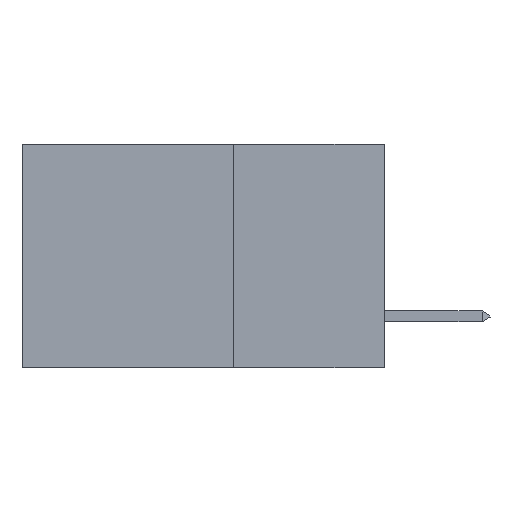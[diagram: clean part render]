
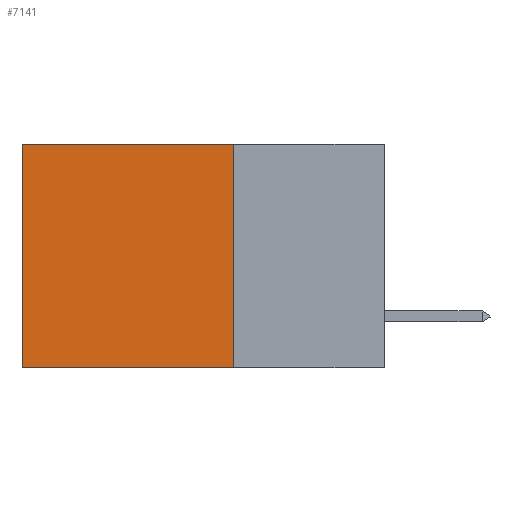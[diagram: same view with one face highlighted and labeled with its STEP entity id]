
A CAD part, left-side view. The second image highlights one B-rep face of the part: STEP entity #7141.
In plain terms, the highlighted planar face has unit normal (-1, 0, 0).
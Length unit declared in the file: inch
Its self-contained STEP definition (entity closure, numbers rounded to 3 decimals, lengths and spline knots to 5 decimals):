
#750 = DIRECTION ( 'NONE',  ( 0., 1., 0. ) ) ;
#767 = CARTESIAN_POINT ( 'NONE',  ( 0.2875, 0.25, 0. ) ) ;
#786 = CARTESIAN_POINT ( 'NONE',  ( 0.2875, 0.25, -0.37 ) ) ;
#958 = CARTESIAN_POINT ( 'NONE',  ( 0.2875, 0.25, -0.37 ) ) ;
#1591 = ORIENTED_EDGE ( 'NONE', *, *, #9707, .F. ) ;
#1870 = CARTESIAN_POINT ( 'NONE',  ( 0.2875, 0.25, 0. ) ) ;
#2051 = DIRECTION ( 'NONE',  ( 0., 1., 0. ) ) ;
#2283 = CARTESIAN_POINT ( 'NONE',  ( 0.2875, 0.6, -0.37 ) ) ;
#2964 = EDGE_LOOP ( 'NONE', ( #13483, #3197, #1591, #3851 ) ) ;
#3197 = ORIENTED_EDGE ( 'NONE', *, *, #10317, .F. ) ;
#3851 = ORIENTED_EDGE ( 'NONE', *, *, #4034, .T. ) ;
#4034 = EDGE_CURVE ( 'NONE', #12528, #10254, #13671, .T. ) ;
#5376 = VECTOR ( 'NONE', #750, 39.37008 ) ;
#5747 = DIRECTION ( 'NONE',  ( 0., 0., -1. ) ) ;
#6283 = VECTOR ( 'NONE', #5747, 39.37008 ) ;
#7141 = ADVANCED_FACE ( 'NONE', ( #13557 ), #7503, .F. ) ;
#7503 = PLANE ( 'NONE',  #9965 ) ;
#7609 = CARTESIAN_POINT ( 'NONE',  ( 0.2875, 0.6, 0. ) ) ;
#8618 = DIRECTION ( 'NONE',  ( 1., 0., 0. ) ) ;
#9707 = EDGE_CURVE ( 'NONE', #12528, #14511, #9827, .T. ) ;
#9806 = DIRECTION ( 'NONE',  ( 0., 0., -1. ) ) ;
#9827 = LINE ( 'NONE', #1870, #6283 ) ;
#9860 = CARTESIAN_POINT ( 'NONE',  ( 0.2875, 0.25, 0. ) ) ;
#9965 = AXIS2_PLACEMENT_3D ( 'NONE', #9860, #8618, #9806 ) ;
#10254 = VERTEX_POINT ( 'NONE', #15386 ) ;
#10306 = VECTOR ( 'NONE', #14868, 39.37008 ) ;
#10317 = EDGE_CURVE ( 'NONE', #14511, #14085, #13210, .T. ) ;
#11919 = VECTOR ( 'NONE', #2051, 39.37008 ) ;
#12424 = EDGE_CURVE ( 'NONE', #10254, #14085, #13897, .T. ) ;
#12528 = VERTEX_POINT ( 'NONE', #767 ) ;
#13210 = LINE ( 'NONE', #786, #11919 ) ;
#13483 = ORIENTED_EDGE ( 'NONE', *, *, #12424, .T. ) ;
#13557 = FACE_OUTER_BOUND ( 'NONE', #2964, .T. ) ;
#13671 = LINE ( 'NONE', #15135, #5376 ) ;
#13897 = LINE ( 'NONE', #7609, #10306 ) ;
#14085 = VERTEX_POINT ( 'NONE', #2283 ) ;
#14511 = VERTEX_POINT ( 'NONE', #958 ) ;
#14868 = DIRECTION ( 'NONE',  ( 0., 0., -1. ) ) ;
#15135 = CARTESIAN_POINT ( 'NONE',  ( 0.2875, 0.25, 0. ) ) ;
#15386 = CARTESIAN_POINT ( 'NONE',  ( 0.2875, 0.6, 0. ) ) ;
